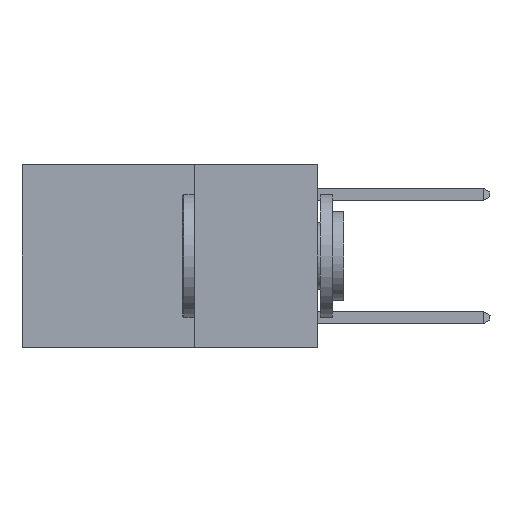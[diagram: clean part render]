
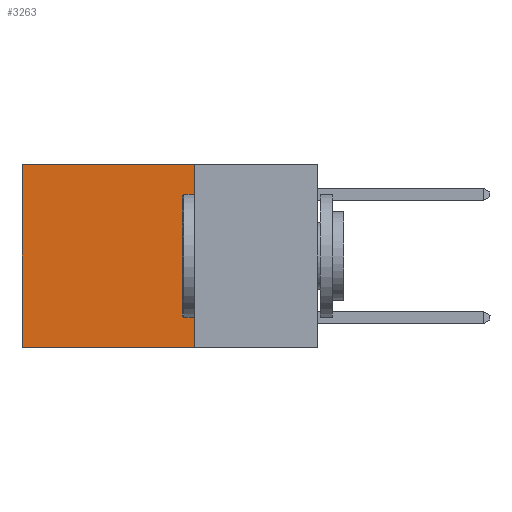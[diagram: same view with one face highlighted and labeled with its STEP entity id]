
A CAD part, left-side view. The second image highlights one B-rep face of the part: STEP entity #3263.
In plain terms, the highlighted planar face has unit normal (-1, 0, 0).
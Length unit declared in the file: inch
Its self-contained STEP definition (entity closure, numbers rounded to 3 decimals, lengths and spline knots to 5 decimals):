
#619 = CARTESIAN_POINT ( 'NONE',  ( 0.2625, 0.25, 0. ) ) ;
#656 = CARTESIAN_POINT ( 'NONE',  ( 0.2625, 0.6, -0.37 ) ) ;
#1428 = VERTEX_POINT ( 'NONE', #656 ) ;
#1490 = CARTESIAN_POINT ( 'NONE',  ( 0.2625, 0.25, -0.37 ) ) ;
#1933 = LINE ( 'NONE', #12832, #5861 ) ;
#1962 = VERTEX_POINT ( 'NONE', #2665 ) ;
#2070 = VECTOR ( 'NONE', #10543, 39.37008 ) ;
#2613 = LINE ( 'NONE', #13451, #2070 ) ;
#2665 = CARTESIAN_POINT ( 'NONE',  ( 0.2625, 0.6, 0. ) ) ;
#3252 = CARTESIAN_POINT ( 'NONE',  ( 0.2625, 0.25, 0. ) ) ;
#3263 = ADVANCED_FACE ( 'NONE', ( #8772 ), #16850, .F. ) ;
#5005 = DIRECTION ( 'NONE',  ( 0., 0., -1. ) ) ;
#5706 = EDGE_LOOP ( 'NONE', ( #8190, #16475, #13444, #17866 ) ) ;
#5861 = VECTOR ( 'NONE', #11373, 39.37008 ) ;
#7400 = DIRECTION ( 'NONE',  ( 0., 1., 0. ) ) ;
#8190 = ORIENTED_EDGE ( 'NONE', *, *, #14762, .T. ) ;
#8244 = VECTOR ( 'NONE', #7400, 39.37008 ) ;
#8772 = FACE_OUTER_BOUND ( 'NONE', #5706, .T. ) ;
#8845 = VERTEX_POINT ( 'NONE', #619 ) ;
#9134 = LINE ( 'NONE', #13442, #16943 ) ;
#9173 = LINE ( 'NONE', #10296, #8244 ) ;
#10113 = AXIS2_PLACEMENT_3D ( 'NONE', #3252, #13927, #5005 ) ;
#10296 = CARTESIAN_POINT ( 'NONE',  ( 0.2625, 0.25, -0.37 ) ) ;
#10543 = DIRECTION ( 'NONE',  ( 0., 1., 0. ) ) ;
#11373 = DIRECTION ( 'NONE',  ( 0., 0., -1. ) ) ;
#12832 = CARTESIAN_POINT ( 'NONE',  ( 0.2625, 0.6, 0. ) ) ;
#13442 = CARTESIAN_POINT ( 'NONE',  ( 0.2625, 0.25, 0. ) ) ;
#13444 = ORIENTED_EDGE ( 'NONE', *, *, #15064, .F. ) ;
#13451 = CARTESIAN_POINT ( 'NONE',  ( 0.2625, 0.25, 0. ) ) ;
#13927 = DIRECTION ( 'NONE',  ( 1., 0., 0. ) ) ;
#14332 = EDGE_CURVE ( 'NONE', #17925, #1428, #9173, .T. ) ;
#14762 = EDGE_CURVE ( 'NONE', #1962, #1428, #1933, .T. ) ;
#14955 = DIRECTION ( 'NONE',  ( 0., 0., -1. ) ) ;
#15064 = EDGE_CURVE ( 'NONE', #8845, #17925, #9134, .T. ) ;
#16475 = ORIENTED_EDGE ( 'NONE', *, *, #14332, .F. ) ;
#16850 = PLANE ( 'NONE',  #10113 ) ;
#16943 = VECTOR ( 'NONE', #14955, 39.37008 ) ;
#17866 = ORIENTED_EDGE ( 'NONE', *, *, #19455, .T. ) ;
#17925 = VERTEX_POINT ( 'NONE', #1490 ) ;
#19455 = EDGE_CURVE ( 'NONE', #8845, #1962, #2613, .T. ) ;
